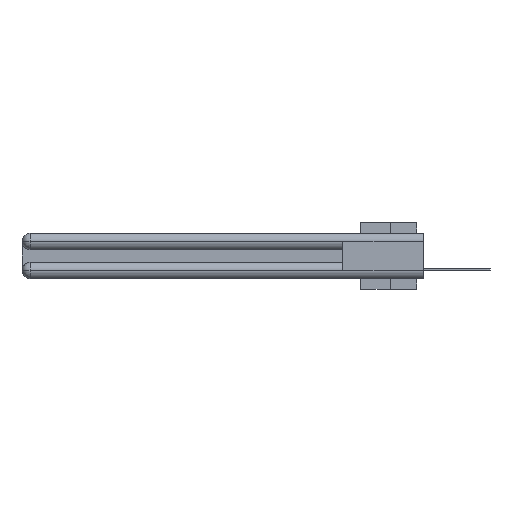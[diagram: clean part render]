
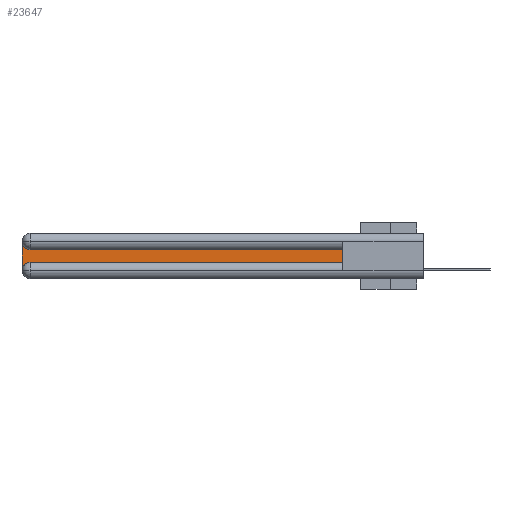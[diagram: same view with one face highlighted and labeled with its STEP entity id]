
A CAD part, left-side view. The second image highlights one B-rep face of the part: STEP entity #23647.
In plain terms, the highlighted planar face has unit normal (-1, 0, 0).
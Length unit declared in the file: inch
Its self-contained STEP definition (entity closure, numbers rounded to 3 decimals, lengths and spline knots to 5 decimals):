
#10 = FACE_OUTER_BOUND ( 'NONE', #21608, .T. ) ;
#149 = DIRECTION ( 'NONE',  ( 0., 0., -1. ) ) ;
#273 = VERTEX_POINT ( 'NONE', #27350 ) ;
#987 = DIRECTION ( 'NONE',  ( 0., 0., -1. ) ) ;
#1220 = ORIENTED_EDGE ( 'NONE', *, *, #31194, .T. ) ;
#2543 = VECTOR ( 'NONE', #987, 39.37008 ) ;
#2651 = CARTESIAN_POINT ( 'NONE',  ( 0.075, 2.94, -0.2775 ) ) ;
#2903 = AXIS2_PLACEMENT_3D ( 'NONE', #25774, #18392, #8790 ) ;
#3020 = AXIS2_PLACEMENT_3D ( 'NONE', #2651, #27741, #149 ) ;
#4152 = DIRECTION ( 'NONE',  ( 0., 1., 0. ) ) ;
#6948 = CARTESIAN_POINT ( 'NONE',  ( 0.075, 3., -0.1225 ) ) ;
#7866 = CARTESIAN_POINT ( 'NONE',  ( 0.075, 0.6, -0.2175 ) ) ;
#8790 = DIRECTION ( 'NONE',  ( 0., 0., -1. ) ) ;
#8820 = CARTESIAN_POINT ( 'NONE',  ( 0.075, 0.6, -0.1225 ) ) ;
#10375 = CARTESIAN_POINT ( 'NONE',  ( 0.075, 2.94, -0.2175 ) ) ;
#11366 = VERTEX_POINT ( 'NONE', #8820 ) ;
#11432 = EDGE_CURVE ( 'NONE', #11366, #273, #14524, .T. ) ;
#13352 = CARTESIAN_POINT ( 'NONE',  ( 0.075, 3., -0.2775 ) ) ;
#14355 = CIRCLE ( 'NONE', #3020, 0.06 ) ;
#14360 = EDGE_CURVE ( 'NONE', #25715, #27690, #29602, .T. ) ;
#14524 = LINE ( 'NONE', #18961, #25359 ) ;
#15186 = LINE ( 'NONE', #26683, #30950 ) ;
#15366 = CARTESIAN_POINT ( 'NONE',  ( 0.075, 0.6, -0.2175 ) ) ;
#15536 = ORIENTED_EDGE ( 'NONE', *, *, #11432, .T. ) ;
#16542 = DIRECTION ( 'NONE',  ( 0., 0., -1. ) ) ;
#16791 = ORIENTED_EDGE ( 'NONE', *, *, #25296, .T. ) ;
#17277 = EDGE_CURVE ( 'NONE', #17771, #18497, #17495, .T. ) ;
#17495 = LINE ( 'NONE', #15366, #30610 ) ;
#17771 = VERTEX_POINT ( 'NONE', #10375 ) ;
#18392 = DIRECTION ( 'NONE',  ( 1., 0., 0. ) ) ;
#18497 = VERTEX_POINT ( 'NONE', #7866 ) ;
#18961 = CARTESIAN_POINT ( 'NONE',  ( 0.075, 0.6, -0.1225 ) ) ;
#19940 = ORIENTED_EDGE ( 'NONE', *, *, #21507, .T. ) ;
#20277 = DIRECTION ( 'NONE',  ( 0., -1., 0. ) ) ;
#21507 = EDGE_CURVE ( 'NONE', #27690, #17771, #14355, .T. ) ;
#21608 = EDGE_LOOP ( 'NONE', ( #15536, #1220, #28303, #19940, #25010, #16791 ) ) ;
#23647 = ADVANCED_FACE ( 'NONE', ( #10 ), #26759, .F. ) ;
#25010 = ORIENTED_EDGE ( 'NONE', *, *, #17277, .T. ) ;
#25296 = EDGE_CURVE ( 'NONE', #18497, #11366, #15186, .T. ) ;
#25359 = VECTOR ( 'NONE', #4152, 39.37008 ) ;
#25680 = AXIS2_PLACEMENT_3D ( 'NONE', #6948, #26883, #16542 ) ;
#25715 = VERTEX_POINT ( 'NONE', #28466 ) ;
#25774 = CARTESIAN_POINT ( 'NONE',  ( 0.075, 2.94, -0.0625 ) ) ;
#26455 = DIRECTION ( 'NONE',  ( 0., 0., 1. ) ) ;
#26683 = CARTESIAN_POINT ( 'NONE',  ( 0.075, 0.6, -0.2175 ) ) ;
#26759 = PLANE ( 'NONE',  #25680 ) ;
#26883 = DIRECTION ( 'NONE',  ( 1., 0., 0. ) ) ;
#27350 = CARTESIAN_POINT ( 'NONE',  ( 0.075, 2.94, -0.1225 ) ) ;
#27690 = VERTEX_POINT ( 'NONE', #13352 ) ;
#27741 = DIRECTION ( 'NONE',  ( 1., 0., 0. ) ) ;
#28303 = ORIENTED_EDGE ( 'NONE', *, *, #14360, .T. ) ;
#28351 = CARTESIAN_POINT ( 'NONE',  ( 0.075, 3., -0.2175 ) ) ;
#28466 = CARTESIAN_POINT ( 'NONE',  ( 0.075, 3., -0.0625 ) ) ;
#29602 = LINE ( 'NONE', #28351, #2543 ) ;
#30312 = CIRCLE ( 'NONE', #2903, 0.06 ) ;
#30610 = VECTOR ( 'NONE', #20277, 39.37008 ) ;
#30950 = VECTOR ( 'NONE', #26455, 39.37008 ) ;
#31194 = EDGE_CURVE ( 'NONE', #273, #25715, #30312, .T. ) ;
